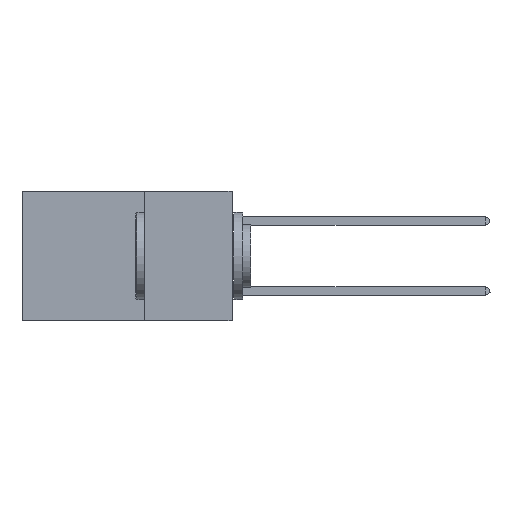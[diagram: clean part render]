
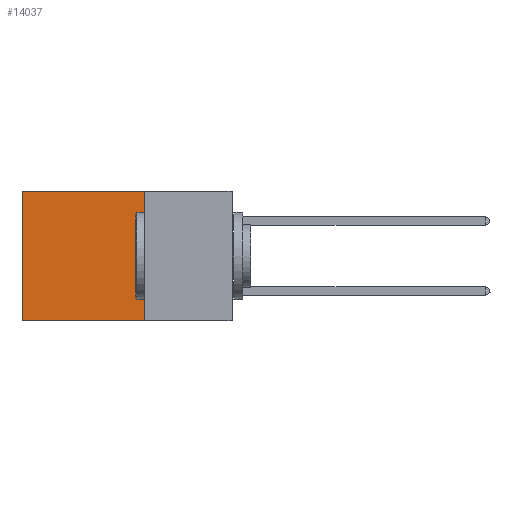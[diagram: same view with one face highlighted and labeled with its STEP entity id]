
A CAD part, left-side view. The second image highlights one B-rep face of the part: STEP entity #14037.
In plain terms, the highlighted planar face has unit normal (-1, 0, 0).
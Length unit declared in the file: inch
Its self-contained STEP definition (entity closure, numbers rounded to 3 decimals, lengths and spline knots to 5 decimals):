
#285 = VERTEX_POINT ( 'NONE', #8869 ) ;
#1236 = CARTESIAN_POINT ( 'NONE',  ( 0.2875, 0.25, 0. ) ) ;
#1386 = VECTOR ( 'NONE', #8627, 39.37008 ) ;
#2003 = VERTEX_POINT ( 'NONE', #11362 ) ;
#2529 = EDGE_CURVE ( 'NONE', #9513, #2003, #16928, .T. ) ;
#2815 = DIRECTION ( 'NONE',  ( 1., 0., 0. ) ) ;
#3484 = CARTESIAN_POINT ( 'NONE',  ( 0.2875, 0.25, 0. ) ) ;
#3756 = DIRECTION ( 'NONE',  ( 0., 1., 0. ) ) ;
#3968 = ORIENTED_EDGE ( 'NONE', *, *, #2529, .T. ) ;
#4142 = EDGE_CURVE ( 'NONE', #5918, #2003, #6718, .T. ) ;
#4235 = AXIS2_PLACEMENT_3D ( 'NONE', #5944, #2815, #6090 ) ;
#5044 = CARTESIAN_POINT ( 'NONE',  ( 0.2875, 0.6, 0. ) ) ;
#5793 = LINE ( 'NONE', #1236, #9516 ) ;
#5918 = VERTEX_POINT ( 'NONE', #11790 ) ;
#5944 = CARTESIAN_POINT ( 'NONE',  ( 0.2875, 0.25, 0. ) ) ;
#6090 = DIRECTION ( 'NONE',  ( 0., 0., -1. ) ) ;
#6718 = LINE ( 'NONE', #19559, #18340 ) ;
#7683 = PLANE ( 'NONE',  #4235 ) ;
#8627 = DIRECTION ( 'NONE',  ( 0., 1., 0. ) ) ;
#8869 = CARTESIAN_POINT ( 'NONE',  ( 0.2875, 0.25, 0. ) ) ;
#9513 = VERTEX_POINT ( 'NONE', #5044 ) ;
#9516 = VECTOR ( 'NONE', #18860, 39.37008 ) ;
#9840 = EDGE_CURVE ( 'NONE', #285, #9513, #17958, .T. ) ;
#11362 = CARTESIAN_POINT ( 'NONE',  ( 0.2875, 0.6, -0.37 ) ) ;
#11790 = CARTESIAN_POINT ( 'NONE',  ( 0.2875, 0.25, -0.37 ) ) ;
#12629 = EDGE_CURVE ( 'NONE', #285, #5918, #5793, .T. ) ;
#13372 = FACE_OUTER_BOUND ( 'NONE', #17618, .T. ) ;
#14037 = ADVANCED_FACE ( 'NONE', ( #13372 ), #7683, .F. ) ;
#15305 = DIRECTION ( 'NONE',  ( 0., 0., -1. ) ) ;
#16150 = ORIENTED_EDGE ( 'NONE', *, *, #4142, .F. ) ;
#16566 = ORIENTED_EDGE ( 'NONE', *, *, #9840, .T. ) ;
#16928 = LINE ( 'NONE', #17497, #19620 ) ;
#17497 = CARTESIAN_POINT ( 'NONE',  ( 0.2875, 0.6, 0. ) ) ;
#17618 = EDGE_LOOP ( 'NONE', ( #3968, #16150, #19399, #16566 ) ) ;
#17958 = LINE ( 'NONE', #3484, #1386 ) ;
#18340 = VECTOR ( 'NONE', #3756, 39.37008 ) ;
#18860 = DIRECTION ( 'NONE',  ( 0., 0., -1. ) ) ;
#19399 = ORIENTED_EDGE ( 'NONE', *, *, #12629, .F. ) ;
#19559 = CARTESIAN_POINT ( 'NONE',  ( 0.2875, 0.25, -0.37 ) ) ;
#19620 = VECTOR ( 'NONE', #15305, 39.37008 ) ;
